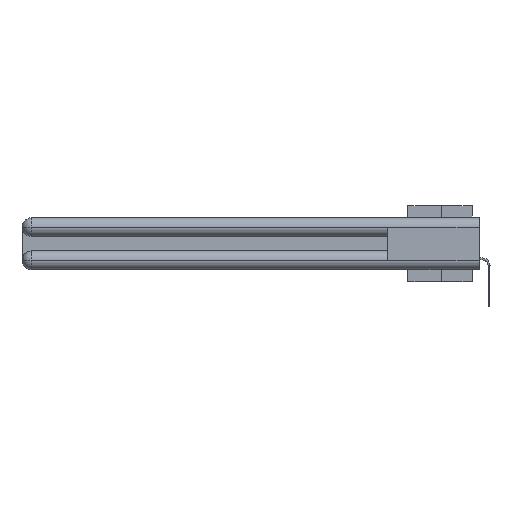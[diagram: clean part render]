
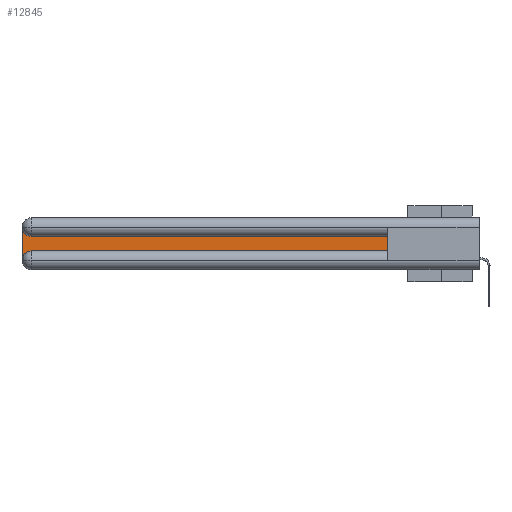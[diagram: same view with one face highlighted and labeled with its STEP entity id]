
A CAD part, left-side view. The second image highlights one B-rep face of the part: STEP entity #12845.
In plain terms, the highlighted planar face has unit normal (-1, 0, 0).
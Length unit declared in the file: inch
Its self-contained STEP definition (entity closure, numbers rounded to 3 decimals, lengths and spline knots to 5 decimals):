
#29 = DIRECTION ( 'NONE',  ( 0., 0., 1. ) ) ;
#863 = LINE ( 'NONE', #8861, #23607 ) ;
#899 = ORIENTED_EDGE ( 'NONE', *, *, #21208, .T. ) ;
#1211 = VERTEX_POINT ( 'NONE', #18845 ) ;
#2165 = VERTEX_POINT ( 'NONE', #19279 ) ;
#3099 = EDGE_CURVE ( 'NONE', #32192, #31300, #9397, .T. ) ;
#3372 = AXIS2_PLACEMENT_3D ( 'NONE', #8686, #22273, #6412 ) ;
#3850 = DIRECTION ( 'NONE',  ( 0., -1., 0. ) ) ;
#4675 = EDGE_CURVE ( 'NONE', #4776, #2165, #863, .T. ) ;
#4776 = VERTEX_POINT ( 'NONE', #15936 ) ;
#4965 = CIRCLE ( 'NONE', #21621, 0.06 ) ;
#5732 = DIRECTION ( 'NONE',  ( 0., 0., -1. ) ) ;
#5759 = DIRECTION ( 'NONE',  ( 0., 0., -1. ) ) ;
#6412 = DIRECTION ( 'NONE',  ( 0., 0., -1. ) ) ;
#6940 = FACE_OUTER_BOUND ( 'NONE', #7931, .T. ) ;
#7852 = VECTOR ( 'NONE', #10247, 39.37008 ) ;
#7931 = EDGE_LOOP ( 'NONE', ( #899, #25059, #29191, #21197, #16069, #13833 ) ) ;
#7999 = EDGE_CURVE ( 'NONE', #31300, #1211, #16351, .T. ) ;
#8686 = CARTESIAN_POINT ( 'NONE',  ( 0.075, 2.94, -0.0625 ) ) ;
#8861 = CARTESIAN_POINT ( 'NONE',  ( 0.075, 3., -0.2175 ) ) ;
#9397 = LINE ( 'NONE', #33218, #29772 ) ;
#10247 = DIRECTION ( 'NONE',  ( 0., 1., 0. ) ) ;
#10598 = AXIS2_PLACEMENT_3D ( 'NONE', #18247, #31282, #12853 ) ;
#11171 = CARTESIAN_POINT ( 'NONE',  ( 0.075, 0.6, -0.2175 ) ) ;
#11926 = VERTEX_POINT ( 'NONE', #18552 ) ;
#12845 = ADVANCED_FACE ( 'NONE', ( #6940 ), #14939, .F. ) ;
#12853 = DIRECTION ( 'NONE',  ( 0., 0., -1. ) ) ;
#12868 = CARTESIAN_POINT ( 'NONE',  ( 0.075, 0.6, -0.1225 ) ) ;
#13833 = ORIENTED_EDGE ( 'NONE', *, *, #7999, .T. ) ;
#14939 = PLANE ( 'NONE',  #10598 ) ;
#15936 = CARTESIAN_POINT ( 'NONE',  ( 0.075, 3., -0.0625 ) ) ;
#16069 = ORIENTED_EDGE ( 'NONE', *, *, #3099, .T. ) ;
#16351 = LINE ( 'NONE', #31838, #20969 ) ;
#18247 = CARTESIAN_POINT ( 'NONE',  ( 0.075, 3., -0.1225 ) ) ;
#18552 = CARTESIAN_POINT ( 'NONE',  ( 0.075, 2.94, -0.1225 ) ) ;
#18845 = CARTESIAN_POINT ( 'NONE',  ( 0.075, 0.6, -0.1225 ) ) ;
#19279 = CARTESIAN_POINT ( 'NONE',  ( 0.075, 3., -0.2775 ) ) ;
#19729 = CARTESIAN_POINT ( 'NONE',  ( 0.075, 2.94, -0.2175 ) ) ;
#20140 = EDGE_CURVE ( 'NONE', #11926, #4776, #27796, .T. ) ;
#20969 = VECTOR ( 'NONE', #29, 39.37008 ) ;
#21197 = ORIENTED_EDGE ( 'NONE', *, *, #30023, .T. ) ;
#21208 = EDGE_CURVE ( 'NONE', #1211, #11926, #22797, .T. ) ;
#21621 = AXIS2_PLACEMENT_3D ( 'NONE', #27325, #22297, #5759 ) ;
#22273 = DIRECTION ( 'NONE',  ( 1., 0., 0. ) ) ;
#22297 = DIRECTION ( 'NONE',  ( 1., 0., 0. ) ) ;
#22797 = LINE ( 'NONE', #12868, #7852 ) ;
#23607 = VECTOR ( 'NONE', #5732, 39.37008 ) ;
#25059 = ORIENTED_EDGE ( 'NONE', *, *, #20140, .T. ) ;
#27325 = CARTESIAN_POINT ( 'NONE',  ( 0.075, 2.94, -0.2775 ) ) ;
#27796 = CIRCLE ( 'NONE', #3372, 0.06 ) ;
#29191 = ORIENTED_EDGE ( 'NONE', *, *, #4675, .T. ) ;
#29772 = VECTOR ( 'NONE', #3850, 39.37008 ) ;
#30023 = EDGE_CURVE ( 'NONE', #2165, #32192, #4965, .T. ) ;
#31282 = DIRECTION ( 'NONE',  ( 1., 0., 0. ) ) ;
#31300 = VERTEX_POINT ( 'NONE', #11171 ) ;
#31838 = CARTESIAN_POINT ( 'NONE',  ( 0.075, 0.6, -0.2175 ) ) ;
#32192 = VERTEX_POINT ( 'NONE', #19729 ) ;
#33218 = CARTESIAN_POINT ( 'NONE',  ( 0.075, 0.6, -0.2175 ) ) ;
